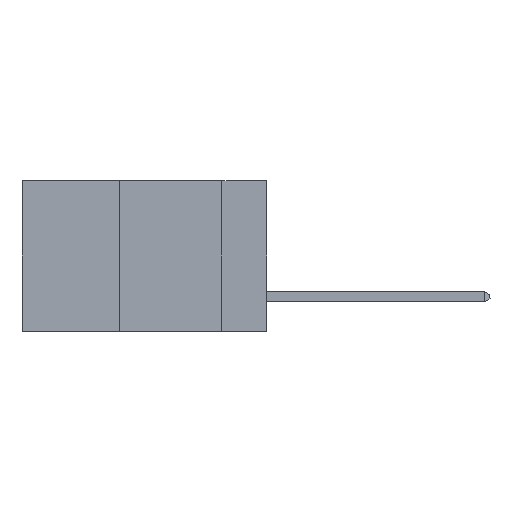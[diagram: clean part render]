
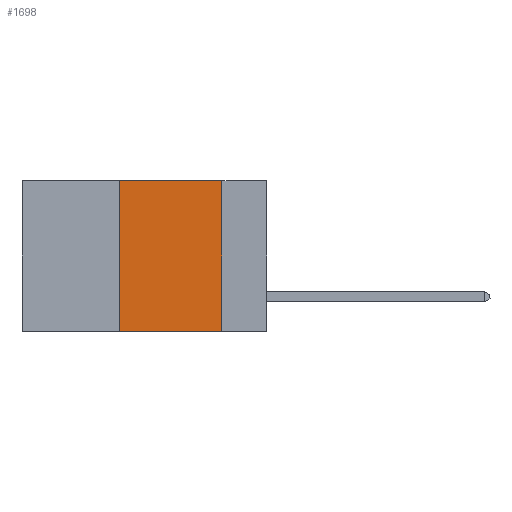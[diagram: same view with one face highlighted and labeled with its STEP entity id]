
A CAD part, left-side view. The second image highlights one B-rep face of the part: STEP entity #1698.
In plain terms, the highlighted planar face has unit normal (-1, 0, 0).
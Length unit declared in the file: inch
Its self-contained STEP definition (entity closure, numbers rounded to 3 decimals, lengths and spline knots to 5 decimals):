
#101 = VECTOR ( 'NONE', #13006, 39.37008 ) ;
#418 = EDGE_CURVE ( 'NONE', #14969, #26775, #14695, .T. ) ;
#613 = CARTESIAN_POINT ( 'NONE',  ( 0., 0.11, -0.37 ) ) ;
#924 = EDGE_CURVE ( 'NONE', #14969, #8924, #7807, .T. ) ;
#1100 = AXIS2_PLACEMENT_3D ( 'NONE', #6559, #14917, #2435 ) ;
#1698 = ADVANCED_FACE ( 'NONE', ( #26171 ), #12810, .F. ) ;
#2269 = VECTOR ( 'NONE', #22783, 39.37008 ) ;
#2435 = DIRECTION ( 'NONE',  ( 0., 0., -1. ) ) ;
#2552 = CARTESIAN_POINT ( 'NONE',  ( 0., 0.11, 0. ) ) ;
#3134 = EDGE_CURVE ( 'NONE', #8924, #6373, #19645, .T. ) ;
#3212 = ORIENTED_EDGE ( 'NONE', *, *, #924, .F. ) ;
#4269 = VECTOR ( 'NONE', #8882, 39.37008 ) ;
#5632 = LINE ( 'NONE', #2552, #101 ) ;
#6373 = VERTEX_POINT ( 'NONE', #20015 ) ;
#6559 = CARTESIAN_POINT ( 'NONE',  ( 0., 0.6, 0. ) ) ;
#7807 = LINE ( 'NONE', #10404, #2269 ) ;
#8658 = VECTOR ( 'NONE', #20404, 39.37008 ) ;
#8882 = DIRECTION ( 'NONE',  ( 0., -1., 0. ) ) ;
#8924 = VERTEX_POINT ( 'NONE', #12717 ) ;
#10070 = ORIENTED_EDGE ( 'NONE', *, *, #22539, .F. ) ;
#10404 = CARTESIAN_POINT ( 'NONE',  ( 0., 0.36, 0. ) ) ;
#11584 = CARTESIAN_POINT ( 'NONE',  ( 0., 0.36, -0.37 ) ) ;
#11930 = EDGE_LOOP ( 'NONE', ( #10070, #19754, #3212, #12969 ) ) ;
#12717 = CARTESIAN_POINT ( 'NONE',  ( 0., 0.36, 0. ) ) ;
#12810 = PLANE ( 'NONE',  #1100 ) ;
#12969 = ORIENTED_EDGE ( 'NONE', *, *, #418, .T. ) ;
#13006 = DIRECTION ( 'NONE',  ( 0., 0., -1. ) ) ;
#14695 = LINE ( 'NONE', #21264, #4269 ) ;
#14917 = DIRECTION ( 'NONE',  ( 1., 0., 0. ) ) ;
#14969 = VERTEX_POINT ( 'NONE', #11584 ) ;
#19645 = LINE ( 'NONE', #26491, #8658 ) ;
#19754 = ORIENTED_EDGE ( 'NONE', *, *, #3134, .F. ) ;
#20015 = CARTESIAN_POINT ( 'NONE',  ( 0., 0.11, 0. ) ) ;
#20404 = DIRECTION ( 'NONE',  ( 0., -1., 0. ) ) ;
#21264 = CARTESIAN_POINT ( 'NONE',  ( 0., 0.6, -0.37 ) ) ;
#22539 = EDGE_CURVE ( 'NONE', #6373, #26775, #5632, .T. ) ;
#22783 = DIRECTION ( 'NONE',  ( 0., 0., 1. ) ) ;
#26171 = FACE_OUTER_BOUND ( 'NONE', #11930, .T. ) ;
#26491 = CARTESIAN_POINT ( 'NONE',  ( 0., 0.6, 0. ) ) ;
#26775 = VERTEX_POINT ( 'NONE', #613 ) ;
